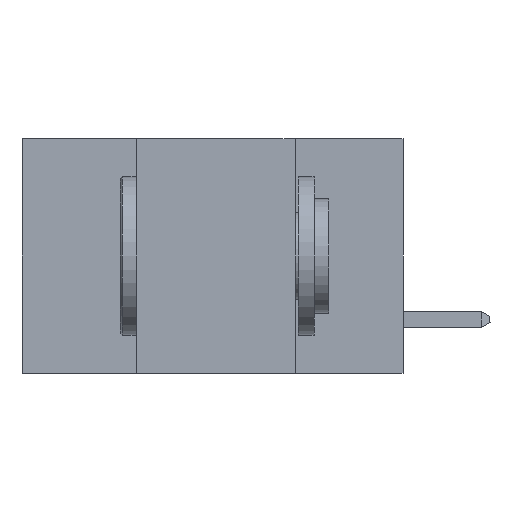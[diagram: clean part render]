
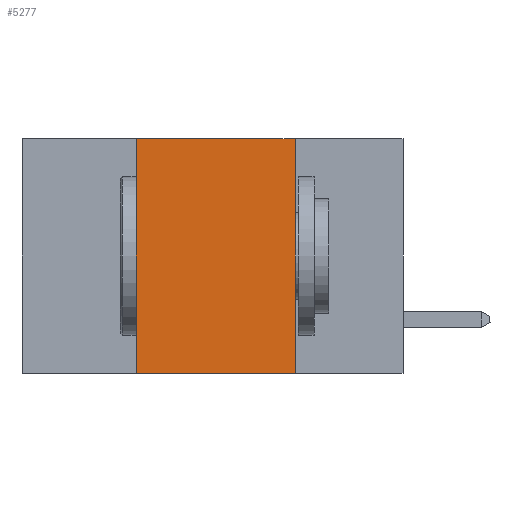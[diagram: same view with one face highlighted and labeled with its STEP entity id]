
A CAD part, left-side view. The second image highlights one B-rep face of the part: STEP entity #5277.
In plain terms, the highlighted planar face has unit normal (-1, 0, 0).
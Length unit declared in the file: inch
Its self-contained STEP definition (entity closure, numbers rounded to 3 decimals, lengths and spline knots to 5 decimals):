
#578 = CARTESIAN_POINT ( 'NONE',  ( 0., 0.42, 0. ) ) ;
#951 = LINE ( 'NONE', #22913, #21847 ) ;
#2110 = DIRECTION ( 'NONE',  ( 0., -1., 0. ) ) ;
#2231 = ORIENTED_EDGE ( 'NONE', *, *, #11060, .F. ) ;
#2516 = ORIENTED_EDGE ( 'NONE', *, *, #3439, .T. ) ;
#3439 = EDGE_CURVE ( 'NONE', #11733, #11013, #13560, .T. ) ;
#3767 = CARTESIAN_POINT ( 'NONE',  ( 0., 0.6, 0. ) ) ;
#4900 = VERTEX_POINT ( 'NONE', #578 ) ;
#5277 = ADVANCED_FACE ( 'NONE', ( #5828 ), #9661, .F. ) ;
#5680 = CARTESIAN_POINT ( 'NONE',  ( 0., 0.42, -0.37 ) ) ;
#5828 = FACE_OUTER_BOUND ( 'NONE', #7006, .T. ) ;
#7006 = EDGE_LOOP ( 'NONE', ( #2231, #11994, #15502, #2516 ) ) ;
#7921 = EDGE_CURVE ( 'NONE', #4900, #17741, #951, .T. ) ;
#9177 = DIRECTION ( 'NONE',  ( 0., 0., 1. ) ) ;
#9661 = PLANE ( 'NONE',  #12727 ) ;
#10030 = CARTESIAN_POINT ( 'NONE',  ( 0., 0.17, 0. ) ) ;
#10687 = CARTESIAN_POINT ( 'NONE',  ( 0., 0.42, 0. ) ) ;
#11013 = VERTEX_POINT ( 'NONE', #11017 ) ;
#11017 = CARTESIAN_POINT ( 'NONE',  ( 0., 0.17, -0.37 ) ) ;
#11060 = EDGE_CURVE ( 'NONE', #17741, #11013, #20003, .T. ) ;
#11313 = DIRECTION ( 'NONE',  ( 1., 0., 0. ) ) ;
#11417 = CARTESIAN_POINT ( 'NONE',  ( 0., 0.6, -0.37 ) ) ;
#11733 = VERTEX_POINT ( 'NONE', #5680 ) ;
#11994 = ORIENTED_EDGE ( 'NONE', *, *, #7921, .F. ) ;
#12727 = AXIS2_PLACEMENT_3D ( 'NONE', #3767, #11313, #17137 ) ;
#13546 = DIRECTION ( 'NONE',  ( 0., -1., 0. ) ) ;
#13560 = LINE ( 'NONE', #11417, #17979 ) ;
#14166 = DIRECTION ( 'NONE',  ( 0., 0., -1. ) ) ;
#15502 = ORIENTED_EDGE ( 'NONE', *, *, #22002, .F. ) ;
#16958 = VECTOR ( 'NONE', #9177, 39.37008 ) ;
#17137 = DIRECTION ( 'NONE',  ( 0., 0., -1. ) ) ;
#17741 = VERTEX_POINT ( 'NONE', #20758 ) ;
#17979 = VECTOR ( 'NONE', #2110, 39.37008 ) ;
#20003 = LINE ( 'NONE', #10030, #20600 ) ;
#20600 = VECTOR ( 'NONE', #14166, 39.37008 ) ;
#20758 = CARTESIAN_POINT ( 'NONE',  ( 0., 0.17, 0. ) ) ;
#21847 = VECTOR ( 'NONE', #13546, 39.37008 ) ;
#21964 = LINE ( 'NONE', #10687, #16958 ) ;
#22002 = EDGE_CURVE ( 'NONE', #11733, #4900, #21964, .T. ) ;
#22913 = CARTESIAN_POINT ( 'NONE',  ( 0., 0.6, 0. ) ) ;
